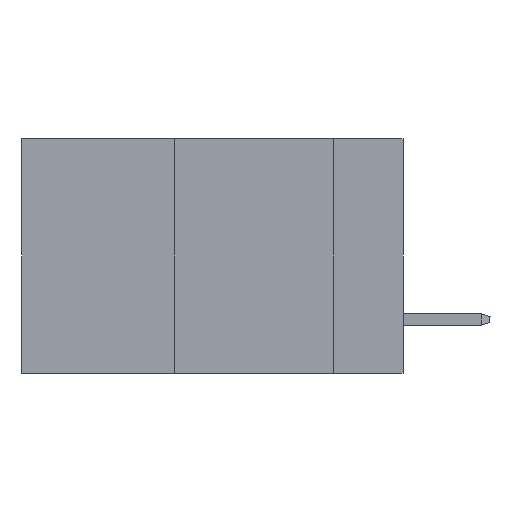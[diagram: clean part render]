
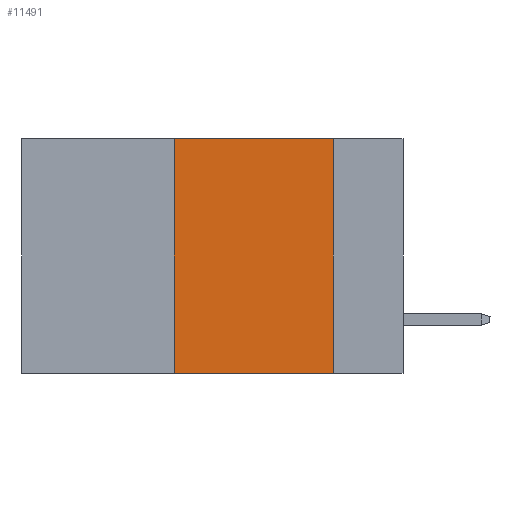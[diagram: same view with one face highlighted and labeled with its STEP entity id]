
A CAD part, left-side view. The second image highlights one B-rep face of the part: STEP entity #11491.
In plain terms, the highlighted planar face has unit normal (-1, 0, 0).
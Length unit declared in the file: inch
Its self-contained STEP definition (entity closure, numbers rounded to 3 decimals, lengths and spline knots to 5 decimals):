
#1336 = LINE ( 'NONE', #21917, #9430 ) ;
#1475 = EDGE_LOOP ( 'NONE', ( #19433, #12706, #20711, #3720 ) ) ;
#1717 = CARTESIAN_POINT ( 'NONE',  ( 0., 0.6, 0. ) ) ;
#2613 = EDGE_CURVE ( 'NONE', #21301, #14562, #1336, .T. ) ;
#3720 = ORIENTED_EDGE ( 'NONE', *, *, #16720, .T. ) ;
#3770 = EDGE_CURVE ( 'NONE', #10641, #16865, #19044, .T. ) ;
#4234 = CARTESIAN_POINT ( 'NONE',  ( 0., 0.36, 0. ) ) ;
#4864 = CARTESIAN_POINT ( 'NONE',  ( 0., 0.11, 0. ) ) ;
#5462 = CARTESIAN_POINT ( 'NONE',  ( 0., 0.6, 0. ) ) ;
#6950 = CARTESIAN_POINT ( 'NONE',  ( 0., 0.36, -0.37 ) ) ;
#7124 = FACE_OUTER_BOUND ( 'NONE', #1475, .T. ) ;
#7361 = PLANE ( 'NONE',  #8464 ) ;
#8380 = VECTOR ( 'NONE', #18239, 39.37008 ) ;
#8464 = AXIS2_PLACEMENT_3D ( 'NONE', #1717, #18223, #9054 ) ;
#9054 = DIRECTION ( 'NONE',  ( 0., 0., -1. ) ) ;
#9430 = VECTOR ( 'NONE', #10493, 39.37008 ) ;
#10493 = DIRECTION ( 'NONE',  ( 0., 0., -1. ) ) ;
#10641 = VERTEX_POINT ( 'NONE', #6950 ) ;
#11491 = ADVANCED_FACE ( 'NONE', ( #7124 ), #7361, .F. ) ;
#11655 = VECTOR ( 'NONE', #20485, 39.37008 ) ;
#12699 = CARTESIAN_POINT ( 'NONE',  ( 0., 0.6, -0.37 ) ) ;
#12706 = ORIENTED_EDGE ( 'NONE', *, *, #22739, .F. ) ;
#13034 = LINE ( 'NONE', #12699, #11655 ) ;
#14562 = VERTEX_POINT ( 'NONE', #19963 ) ;
#14841 = LINE ( 'NONE', #5462, #8380 ) ;
#16720 = EDGE_CURVE ( 'NONE', #10641, #14562, #13034, .T. ) ;
#16865 = VERTEX_POINT ( 'NONE', #22784 ) ;
#18223 = DIRECTION ( 'NONE',  ( 1., 0., 0. ) ) ;
#18239 = DIRECTION ( 'NONE',  ( 0., -1., 0. ) ) ;
#18682 = DIRECTION ( 'NONE',  ( 0., 0., 1. ) ) ;
#19044 = LINE ( 'NONE', #4234, #21546 ) ;
#19433 = ORIENTED_EDGE ( 'NONE', *, *, #2613, .F. ) ;
#19963 = CARTESIAN_POINT ( 'NONE',  ( 0., 0.11, -0.37 ) ) ;
#20485 = DIRECTION ( 'NONE',  ( 0., -1., 0. ) ) ;
#20711 = ORIENTED_EDGE ( 'NONE', *, *, #3770, .F. ) ;
#21301 = VERTEX_POINT ( 'NONE', #4864 ) ;
#21546 = VECTOR ( 'NONE', #18682, 39.37008 ) ;
#21917 = CARTESIAN_POINT ( 'NONE',  ( 0., 0.11, 0. ) ) ;
#22739 = EDGE_CURVE ( 'NONE', #16865, #21301, #14841, .T. ) ;
#22784 = CARTESIAN_POINT ( 'NONE',  ( 0., 0.36, 0. ) ) ;
